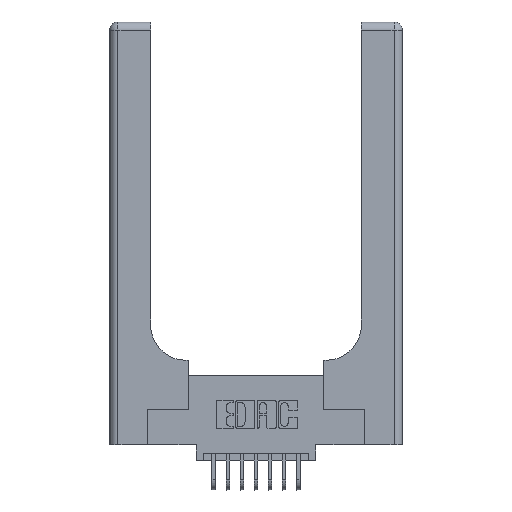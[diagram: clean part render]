
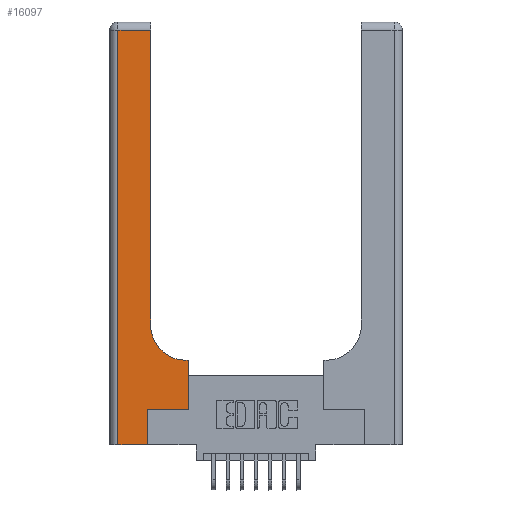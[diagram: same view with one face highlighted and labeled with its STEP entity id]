
A CAD part, top view. The second image highlights one B-rep face of the part: STEP entity #16097.
In plain terms, the highlighted planar face has unit normal (0, 0, 1).
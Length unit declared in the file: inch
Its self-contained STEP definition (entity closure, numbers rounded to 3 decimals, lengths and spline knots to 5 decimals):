
#30 = DIRECTION ( 'NONE',  ( -1., 0., 0. ) ) ;
#133 = EDGE_CURVE ( 'NONE', #7906, #12290, #13353, .T. ) ;
#1026 = LINE ( 'NONE', #4778, #4259 ) ;
#1190 = VERTEX_POINT ( 'NONE', #14909 ) ;
#1229 = VECTOR ( 'NONE', #12005, 39.37008 ) ;
#1327 = CARTESIAN_POINT ( 'NONE',  ( 0.5585, 0.25, 0.37 ) ) ;
#1915 = CARTESIAN_POINT ( 'NONE',  ( 0.2915, 0.85, 0.37 ) ) ;
#2163 = ORIENTED_EDGE ( 'NONE', *, *, #15242, .T. ) ;
#2736 = LINE ( 'NONE', #8256, #9558 ) ;
#2887 = CARTESIAN_POINT ( 'NONE',  ( 0., 0., 0.37 ) ) ;
#3010 = ORIENTED_EDGE ( 'NONE', *, *, #5004, .T. ) ;
#3595 = CARTESIAN_POINT ( 'NONE',  ( 0.5415, 0.85, 0.37 ) ) ;
#4259 = VECTOR ( 'NONE', #6199, 39.37008 ) ;
#4778 = CARTESIAN_POINT ( 'NONE',  ( 0.269, 0., 0.37 ) ) ;
#4940 = ORIENTED_EDGE ( 'NONE', *, *, #13999, .T. ) ;
#4973 = DIRECTION ( 'NONE',  ( 1., 0., 0. ) ) ;
#5004 = EDGE_CURVE ( 'NONE', #12052, #11353, #14838, .T. ) ;
#5325 = CARTESIAN_POINT ( 'NONE',  ( 0.269, 0., 0.37 ) ) ;
#5454 = EDGE_CURVE ( 'NONE', #1190, #6993, #13051, .T. ) ;
#5466 = EDGE_LOOP ( 'NONE', ( #4940, #8602, #8992, #15812, #2163, #16213, #13235, #16614, #3010 ) ) ;
#5969 = FACE_OUTER_BOUND ( 'NONE', #5466, .T. ) ;
#6199 = DIRECTION ( 'NONE',  ( 0., 1., 0. ) ) ;
#6740 = CARTESIAN_POINT ( 'NONE',  ( 0.2915, 2.94, 0.37 ) ) ;
#6800 = DIRECTION ( 'NONE',  ( 1., 0., 0. ) ) ;
#6822 = CARTESIAN_POINT ( 'NONE',  ( 0.269, 0.25, 0.37 ) ) ;
#6946 = CARTESIAN_POINT ( 'NONE',  ( 0., 3., 0.37 ) ) ;
#6952 = CARTESIAN_POINT ( 'NONE',  ( 0.06, 0., 0.37 ) ) ;
#6993 = VERTEX_POINT ( 'NONE', #6952 ) ;
#7408 = CARTESIAN_POINT ( 'NONE',  ( 0.06, 3., 0.37 ) ) ;
#7771 = VECTOR ( 'NONE', #10388, 39.37008 ) ;
#7906 = VERTEX_POINT ( 'NONE', #13138 ) ;
#7992 = EDGE_CURVE ( 'NONE', #10101, #12052, #11986, .T. ) ;
#8148 = DIRECTION ( 'NONE',  ( 0., 1., 0. ) ) ;
#8256 = CARTESIAN_POINT ( 'NONE',  ( 0.5585, 0.25, 0.37 ) ) ;
#8312 = DIRECTION ( 'NONE',  ( 0., 0., -1. ) ) ;
#8592 = LINE ( 'NONE', #9067, #7771 ) ;
#8602 = ORIENTED_EDGE ( 'NONE', *, *, #13829, .T. ) ;
#8992 = ORIENTED_EDGE ( 'NONE', *, *, #5454, .T. ) ;
#9067 = CARTESIAN_POINT ( 'NONE',  ( 0., 2.94, 0.37 ) ) ;
#9071 = CARTESIAN_POINT ( 'NONE',  ( 0.5415, 0.6, 0.37 ) ) ;
#9543 = VECTOR ( 'NONE', #6800, 39.37008 ) ;
#9558 = VECTOR ( 'NONE', #12137, 39.37008 ) ;
#9595 = AXIS2_PLACEMENT_3D ( 'NONE', #6946, #8312, #30 ) ;
#10101 = VERTEX_POINT ( 'NONE', #13728 ) ;
#10388 = DIRECTION ( 'NONE',  ( -1., 0., 0. ) ) ;
#10715 = LINE ( 'NONE', #2887, #17084 ) ;
#10732 = CARTESIAN_POINT ( 'NONE',  ( 0.2915, 0.6, 0.37 ) ) ;
#11096 = VERTEX_POINT ( 'NONE', #5325 ) ;
#11211 = EDGE_CURVE ( 'NONE', #6993, #11096, #10715, .T. ) ;
#11353 = VERTEX_POINT ( 'NONE', #1915 ) ;
#11615 = VERTEX_POINT ( 'NONE', #6740 ) ;
#11986 = LINE ( 'NONE', #10732, #1229 ) ;
#12005 = DIRECTION ( 'NONE',  ( -1., 0., 0. ) ) ;
#12052 = VERTEX_POINT ( 'NONE', #9071 ) ;
#12137 = DIRECTION ( 'NONE',  ( 0., 1., 0. ) ) ;
#12290 = VERTEX_POINT ( 'NONE', #1327 ) ;
#12617 = LINE ( 'NONE', #14553, #15200 ) ;
#12935 = DIRECTION ( 'NONE',  ( 0., 0., -1. ) ) ;
#13051 = LINE ( 'NONE', #7408, #15627 ) ;
#13138 = CARTESIAN_POINT ( 'NONE',  ( 0.269, 0.25, 0.37 ) ) ;
#13235 = ORIENTED_EDGE ( 'NONE', *, *, #16078, .T. ) ;
#13353 = LINE ( 'NONE', #6822, #9543 ) ;
#13522 = DIRECTION ( 'NONE',  ( 1., 0., 0. ) ) ;
#13728 = CARTESIAN_POINT ( 'NONE',  ( 0.5585, 0.6, 0.37 ) ) ;
#13829 = EDGE_CURVE ( 'NONE', #11615, #1190, #8592, .T. ) ;
#13848 = DIRECTION ( 'NONE',  ( 0., -1., 0. ) ) ;
#13999 = EDGE_CURVE ( 'NONE', #11353, #11615, #12617, .T. ) ;
#14049 = AXIS2_PLACEMENT_3D ( 'NONE', #3595, #12935, #4973 ) ;
#14553 = CARTESIAN_POINT ( 'NONE',  ( 0.2915, 3., 0.37 ) ) ;
#14838 = CIRCLE ( 'NONE', #14049, 0.25 ) ;
#14909 = CARTESIAN_POINT ( 'NONE',  ( 0.06, 2.94, 0.37 ) ) ;
#15200 = VECTOR ( 'NONE', #8148, 39.37008 ) ;
#15242 = EDGE_CURVE ( 'NONE', #11096, #7906, #1026, .T. ) ;
#15627 = VECTOR ( 'NONE', #13848, 39.37008 ) ;
#15812 = ORIENTED_EDGE ( 'NONE', *, *, #11211, .T. ) ;
#15991 = PLANE ( 'NONE',  #9595 ) ;
#16078 = EDGE_CURVE ( 'NONE', #12290, #10101, #2736, .T. ) ;
#16097 = ADVANCED_FACE ( 'NONE', ( #5969 ), #15991, .F. ) ;
#16213 = ORIENTED_EDGE ( 'NONE', *, *, #133, .T. ) ;
#16614 = ORIENTED_EDGE ( 'NONE', *, *, #7992, .T. ) ;
#17084 = VECTOR ( 'NONE', #13522, 39.37008 ) ;
